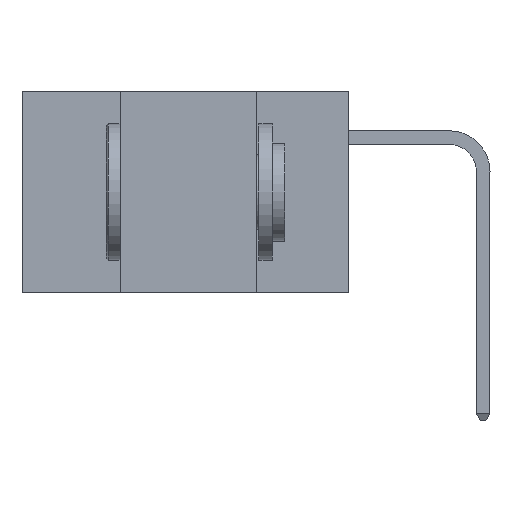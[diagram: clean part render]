
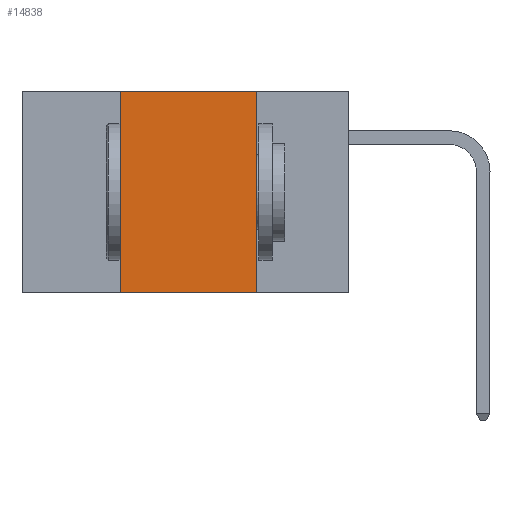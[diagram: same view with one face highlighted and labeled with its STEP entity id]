
A CAD part, left-side view. The second image highlights one B-rep face of the part: STEP entity #14838.
In plain terms, the highlighted planar face has unit normal (-1, 0, 0).
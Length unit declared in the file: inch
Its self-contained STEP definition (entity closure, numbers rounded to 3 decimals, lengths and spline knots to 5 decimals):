
#90 = CARTESIAN_POINT ( 'NONE',  ( 0., 0.42, 0. ) ) ;
#911 = CARTESIAN_POINT ( 'NONE',  ( 0., 0.42, -0.37 ) ) ;
#1114 = CARTESIAN_POINT ( 'NONE',  ( 0., 0.17, 0. ) ) ;
#1491 = CARTESIAN_POINT ( 'NONE',  ( 0., 0.42, 0. ) ) ;
#2129 = EDGE_CURVE ( 'NONE', #4071, #13381, #2155, .T. ) ;
#2155 = LINE ( 'NONE', #90, #17189 ) ;
#2345 = VECTOR ( 'NONE', #19389, 39.37008 ) ;
#3734 = LINE ( 'NONE', #1114, #6770 ) ;
#4071 = VERTEX_POINT ( 'NONE', #911 ) ;
#4970 = ORIENTED_EDGE ( 'NONE', *, *, #2129, .F. ) ;
#6770 = VECTOR ( 'NONE', #18914, 39.37008 ) ;
#9187 = ORIENTED_EDGE ( 'NONE', *, *, #26219, .F. ) ;
#9840 = DIRECTION ( 'NONE',  ( 0., 0., -1. ) ) ;
#10080 = VERTEX_POINT ( 'NONE', #13925 ) ;
#10765 = DIRECTION ( 'NONE',  ( 0., 0., 1. ) ) ;
#11845 = CARTESIAN_POINT ( 'NONE',  ( 0., 0.6, 0. ) ) ;
#12102 = EDGE_CURVE ( 'NONE', #13381, #19545, #22877, .T. ) ;
#13381 = VERTEX_POINT ( 'NONE', #1491 ) ;
#13427 = ORIENTED_EDGE ( 'NONE', *, *, #26195, .T. ) ;
#13900 = AXIS2_PLACEMENT_3D ( 'NONE', #11845, #16166, #9840 ) ;
#13925 = CARTESIAN_POINT ( 'NONE',  ( 0., 0.17, -0.37 ) ) ;
#14080 = DIRECTION ( 'NONE',  ( 0., -1., 0. ) ) ;
#14838 = ADVANCED_FACE ( 'NONE', ( #19300 ), #16053, .F. ) ;
#16053 = PLANE ( 'NONE',  #13900 ) ;
#16166 = DIRECTION ( 'NONE',  ( 1., 0., 0. ) ) ;
#17189 = VECTOR ( 'NONE', #10765, 39.37008 ) ;
#18641 = EDGE_LOOP ( 'NONE', ( #9187, #24147, #4970, #13427 ) ) ;
#18914 = DIRECTION ( 'NONE',  ( 0., 0., -1. ) ) ;
#19300 = FACE_OUTER_BOUND ( 'NONE', #18641, .T. ) ;
#19389 = DIRECTION ( 'NONE',  ( 0., -1., 0. ) ) ;
#19545 = VERTEX_POINT ( 'NONE', #26684 ) ;
#20917 = CARTESIAN_POINT ( 'NONE',  ( 0., 0.6, 0. ) ) ;
#22877 = LINE ( 'NONE', #20917, #26600 ) ;
#24147 = ORIENTED_EDGE ( 'NONE', *, *, #12102, .F. ) ;
#25449 = CARTESIAN_POINT ( 'NONE',  ( 0., 0.6, -0.37 ) ) ;
#25498 = LINE ( 'NONE', #25449, #2345 ) ;
#26195 = EDGE_CURVE ( 'NONE', #4071, #10080, #25498, .T. ) ;
#26219 = EDGE_CURVE ( 'NONE', #19545, #10080, #3734, .T. ) ;
#26600 = VECTOR ( 'NONE', #14080, 39.37008 ) ;
#26684 = CARTESIAN_POINT ( 'NONE',  ( 0., 0.17, 0. ) ) ;
